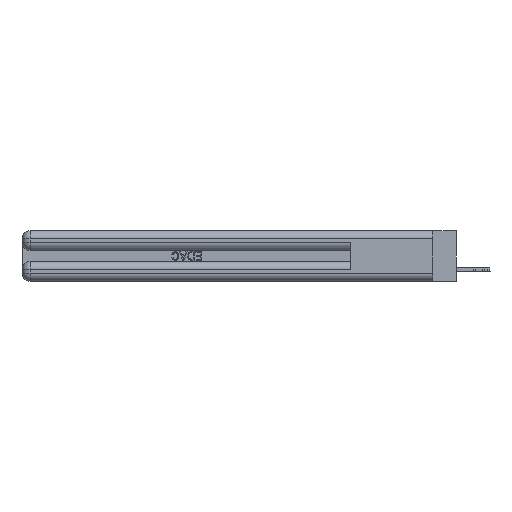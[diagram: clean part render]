
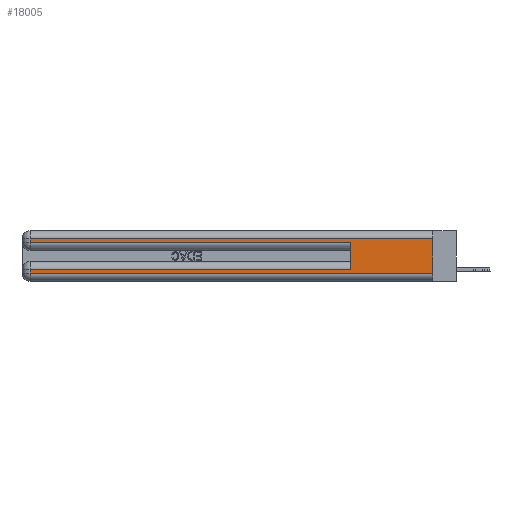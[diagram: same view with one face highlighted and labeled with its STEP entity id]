
A CAD part, left-side view. The second image highlights one B-rep face of the part: STEP entity #18005.
In plain terms, the highlighted planar face has unit normal (-1, 0, 0).
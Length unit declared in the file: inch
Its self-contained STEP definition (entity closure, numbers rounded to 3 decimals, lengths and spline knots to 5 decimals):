
#61 = LINE ( 'NONE', #17972, #37795 ) ;
#434 = LINE ( 'NONE', #43845, #45598 ) ;
#441 = FACE_OUTER_BOUND ( 'NONE', #32285, .T. ) ;
#1212 = DIRECTION ( 'NONE',  ( 0., 0., -1. ) ) ;
#1474 = VERTEX_POINT ( 'NONE', #12642 ) ;
#1509 = VECTOR ( 'NONE', #30247, 39.37008 ) ;
#2528 = CARTESIAN_POINT ( 'NONE',  ( 0., 0., 0.06 ) ) ;
#3785 = EDGE_CURVE ( 'NONE', #33920, #34382, #61, .T. ) ;
#4086 = AXIS2_PLACEMENT_3D ( 'NONE', #32040, #25314, #24869 ) ;
#4227 = EDGE_CURVE ( 'NONE', #23296, #1474, #13230, .T. ) ;
#4684 = ORIENTED_EDGE ( 'NONE', *, *, #18189, .T. ) ;
#5143 = VERTEX_POINT ( 'NONE', #46645 ) ;
#5175 = CARTESIAN_POINT ( 'NONE',  ( 0., 0., 0.31 ) ) ;
#5537 = CARTESIAN_POINT ( 'NONE',  ( 0., 0., 0.285 ) ) ;
#5893 = DIRECTION ( 'NONE',  ( 0., -1., 0. ) ) ;
#8981 = CARTESIAN_POINT ( 'NONE',  ( 0., 2.94, 0.37 ) ) ;
#9734 = ORIENTED_EDGE ( 'NONE', *, *, #43407, .T. ) ;
#10494 = PLANE ( 'NONE',  #4086 ) ;
#12528 = ORIENTED_EDGE ( 'NONE', *, *, #30957, .F. ) ;
#12642 = CARTESIAN_POINT ( 'NONE',  ( 0., 2.94, 0.285 ) ) ;
#13230 = LINE ( 'NONE', #19496, #41748 ) ;
#13929 = CARTESIAN_POINT ( 'NONE',  ( 0., 0., 0.085 ) ) ;
#15142 = LINE ( 'NONE', #8981, #25993 ) ;
#17972 = CARTESIAN_POINT ( 'NONE',  ( 0., 0., 0.37 ) ) ;
#18005 = ADVANCED_FACE ( 'NONE', ( #441 ), #10494, .F. ) ;
#18189 = EDGE_CURVE ( 'NONE', #33920, #23296, #25601, .T. ) ;
#19496 = CARTESIAN_POINT ( 'NONE',  ( 0., 2.94, 0.37 ) ) ;
#20180 = DIRECTION ( 'NONE',  ( 0., 0., -1. ) ) ;
#20710 = ORIENTED_EDGE ( 'NONE', *, *, #37644, .T. ) ;
#21593 = LINE ( 'NONE', #13929, #43841 ) ;
#23296 = VERTEX_POINT ( 'NONE', #32072 ) ;
#23593 = VERTEX_POINT ( 'NONE', #24070 ) ;
#24070 = CARTESIAN_POINT ( 'NONE',  ( 0., 0.6, 0.285 ) ) ;
#24297 = EDGE_CURVE ( 'NONE', #5143, #34382, #29022, .T. ) ;
#24538 = CARTESIAN_POINT ( 'NONE',  ( 0., 0.6, 0.085 ) ) ;
#24869 = DIRECTION ( 'NONE',  ( 0., 0., -1. ) ) ;
#25314 = DIRECTION ( 'NONE',  ( 1., 0., 0. ) ) ;
#25601 = LINE ( 'NONE', #41109, #1509 ) ;
#25993 = VECTOR ( 'NONE', #20180, 39.37008 ) ;
#26227 = CARTESIAN_POINT ( 'NONE',  ( 0., 2.94, 0.085 ) ) ;
#26278 = ORIENTED_EDGE ( 'NONE', *, *, #4227, .T. ) ;
#27055 = VECTOR ( 'NONE', #34810, 39.37008 ) ;
#29022 = LINE ( 'NONE', #2528, #45566 ) ;
#29126 = DIRECTION ( 'NONE',  ( 0., 0., -1. ) ) ;
#30247 = DIRECTION ( 'NONE',  ( 0., 1., 0. ) ) ;
#30957 = EDGE_CURVE ( 'NONE', #35217, #23593, #434, .T. ) ;
#31776 = VERTEX_POINT ( 'NONE', #26227 ) ;
#32040 = CARTESIAN_POINT ( 'NONE',  ( 0., 0., 0.37 ) ) ;
#32072 = CARTESIAN_POINT ( 'NONE',  ( 0., 2.94, 0.31 ) ) ;
#32108 = DIRECTION ( 'NONE',  ( 0., 1., 0. ) ) ;
#32285 = EDGE_LOOP ( 'NONE', ( #46264, #4684, #26278, #9734, #12528, #46045, #20710, #40933 ) ) ;
#33920 = VERTEX_POINT ( 'NONE', #5175 ) ;
#34382 = VERTEX_POINT ( 'NONE', #44152 ) ;
#34810 = DIRECTION ( 'NONE',  ( 0., -1., 0. ) ) ;
#35217 = VERTEX_POINT ( 'NONE', #24538 ) ;
#37644 = EDGE_CURVE ( 'NONE', #31776, #5143, #15142, .T. ) ;
#37795 = VECTOR ( 'NONE', #29126, 39.37008 ) ;
#40508 = DIRECTION ( 'NONE',  ( 0., 0., 1. ) ) ;
#40800 = LINE ( 'NONE', #5537, #27055 ) ;
#40933 = ORIENTED_EDGE ( 'NONE', *, *, #24297, .T. ) ;
#41109 = CARTESIAN_POINT ( 'NONE',  ( 0., 0., 0.31 ) ) ;
#41561 = EDGE_CURVE ( 'NONE', #35217, #31776, #21593, .T. ) ;
#41748 = VECTOR ( 'NONE', #1212, 39.37008 ) ;
#43407 = EDGE_CURVE ( 'NONE', #1474, #23593, #40800, .T. ) ;
#43841 = VECTOR ( 'NONE', #32108, 39.37008 ) ;
#43845 = CARTESIAN_POINT ( 'NONE',  ( 0., 0.6, 0.145 ) ) ;
#44152 = CARTESIAN_POINT ( 'NONE',  ( 0., 0., 0.06 ) ) ;
#45566 = VECTOR ( 'NONE', #5893, 39.37008 ) ;
#45598 = VECTOR ( 'NONE', #40508, 39.37008 ) ;
#46045 = ORIENTED_EDGE ( 'NONE', *, *, #41561, .T. ) ;
#46264 = ORIENTED_EDGE ( 'NONE', *, *, #3785, .F. ) ;
#46645 = CARTESIAN_POINT ( 'NONE',  ( 0., 2.94, 0.06 ) ) ;
